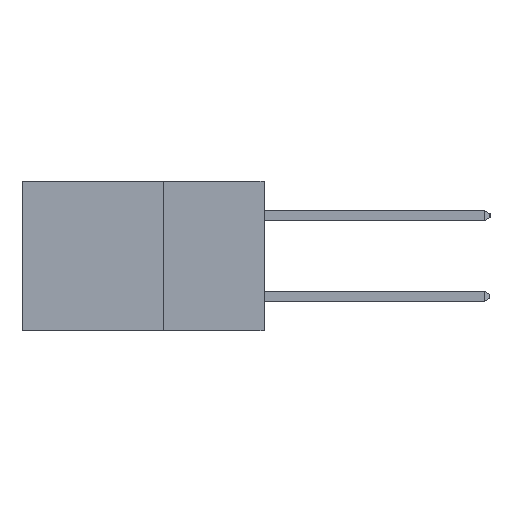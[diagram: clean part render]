
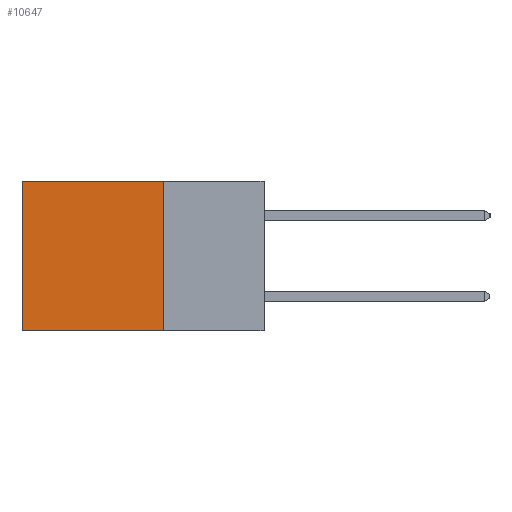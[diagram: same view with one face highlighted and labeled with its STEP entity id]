
A CAD part, left-side view. The second image highlights one B-rep face of the part: STEP entity #10647.
In plain terms, the highlighted planar face has unit normal (-1, 0, 0).
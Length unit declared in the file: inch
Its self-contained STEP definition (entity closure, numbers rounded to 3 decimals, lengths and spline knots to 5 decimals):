
#123 = EDGE_LOOP ( 'NONE', ( #9919, #3258, #1423, #1684 ) ) ;
#648 = CARTESIAN_POINT ( 'NONE',  ( 0.2615, 0.6, 0. ) ) ;
#1423 = ORIENTED_EDGE ( 'NONE', *, *, #9995, .F. ) ;
#1684 = ORIENTED_EDGE ( 'NONE', *, *, #6245, .T. ) ;
#2205 = CARTESIAN_POINT ( 'NONE',  ( 0.2615, 0.6, -0.37 ) ) ;
#2430 = FACE_OUTER_BOUND ( 'NONE', #123, .T. ) ;
#2482 = CARTESIAN_POINT ( 'NONE',  ( 0.2615, 0.25, -0.37 ) ) ;
#2516 = VECTOR ( 'NONE', #9986, 39.37008 ) ;
#2592 = VERTEX_POINT ( 'NONE', #7643 ) ;
#3244 = VERTEX_POINT ( 'NONE', #648 ) ;
#3258 = ORIENTED_EDGE ( 'NONE', *, *, #4958, .F. ) ;
#3309 = VECTOR ( 'NONE', #5168, 39.37008 ) ;
#4048 = CARTESIAN_POINT ( 'NONE',  ( 0.2615, 0.25, -0.37 ) ) ;
#4114 = VERTEX_POINT ( 'NONE', #11005 ) ;
#4306 = AXIS2_PLACEMENT_3D ( 'NONE', #4048, #10734, #11773 ) ;
#4323 = LINE ( 'NONE', #10835, #11584 ) ;
#4958 = EDGE_CURVE ( 'NONE', #4114, #7477, #9271, .T. ) ;
#5168 = DIRECTION ( 'NONE',  ( 0., 0., -1. ) ) ;
#5438 = DIRECTION ( 'NONE',  ( 0., 1., 0. ) ) ;
#5508 = CARTESIAN_POINT ( 'NONE',  ( 0.2615, 0.25, 0. ) ) ;
#5777 = CARTESIAN_POINT ( 'NONE',  ( 0.2615, 0.6, -0.37 ) ) ;
#6144 = VECTOR ( 'NONE', #5438, 39.37008 ) ;
#6245 = EDGE_CURVE ( 'NONE', #2592, #3244, #11952, .T. ) ;
#6952 = LINE ( 'NONE', #2205, #3309 ) ;
#7477 = VERTEX_POINT ( 'NONE', #5777 ) ;
#7643 = CARTESIAN_POINT ( 'NONE',  ( 0.2615, 0.25, 0. ) ) ;
#9271 = LINE ( 'NONE', #2482, #2516 ) ;
#9751 = PLANE ( 'NONE',  #4306 ) ;
#9919 = ORIENTED_EDGE ( 'NONE', *, *, #10371, .T. ) ;
#9986 = DIRECTION ( 'NONE',  ( 0., 1., 0. ) ) ;
#9995 = EDGE_CURVE ( 'NONE', #2592, #4114, #4323, .T. ) ;
#10371 = EDGE_CURVE ( 'NONE', #3244, #7477, #6952, .T. ) ;
#10596 = DIRECTION ( 'NONE',  ( 0., 0., -1. ) ) ;
#10647 = ADVANCED_FACE ( 'NONE', ( #2430 ), #9751, .F. ) ;
#10734 = DIRECTION ( 'NONE',  ( 1., 0., 0. ) ) ;
#10835 = CARTESIAN_POINT ( 'NONE',  ( 0.2615, 0.25, -0.37 ) ) ;
#11005 = CARTESIAN_POINT ( 'NONE',  ( 0.2615, 0.25, -0.37 ) ) ;
#11584 = VECTOR ( 'NONE', #10596, 39.37008 ) ;
#11773 = DIRECTION ( 'NONE',  ( 0., 0., -1. ) ) ;
#11952 = LINE ( 'NONE', #5508, #6144 ) ;
